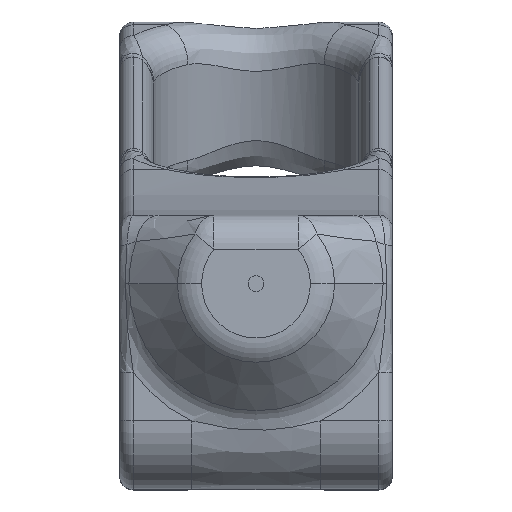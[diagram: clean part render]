
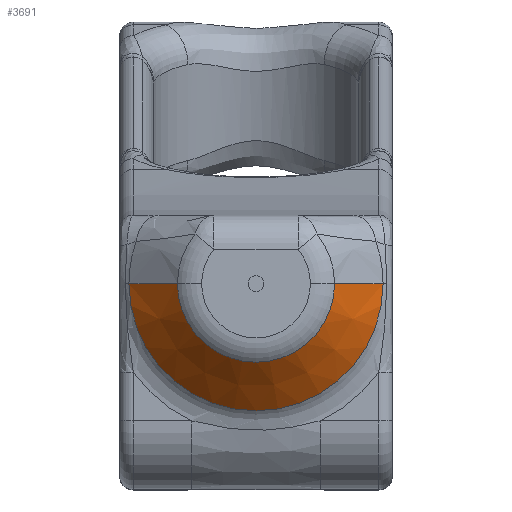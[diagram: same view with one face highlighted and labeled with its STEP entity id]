
A CAD part, top view. The second image highlights one B-rep face of the part: STEP entity #3691.
In plain terms, the highlighted conical face has half-angle 45 degrees and reference radius 5 mm.
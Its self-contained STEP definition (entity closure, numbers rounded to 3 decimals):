
#297 = EDGE_CURVE ( 'NONE', #1811, #1829, #3724, .T. ) ;
#663 = CARTESIAN_POINT ( 'NONE',  ( 0.681, 5., 18.232 ) ) ;
#1029 = DIRECTION ( 'NONE',  ( 0., 0., 1. ) ) ;
#1056 = EDGE_CURVE ( 'NONE', #2212, #2145, #3597, .T. ) ;
#1210 = DIRECTION ( 'NONE',  ( -1., 0., 0. ) ) ;
#1235 = EDGE_CURVE ( 'NONE', #2212, #1811, #2116, .T. ) ;
#1811 = VERTEX_POINT ( 'NONE', #3939 ) ;
#1829 = VERTEX_POINT ( 'NONE', #663 ) ;
#2077 = ORIENTED_EDGE ( 'NONE', *, *, #4556, .T. ) ;
#2116 = CIRCLE ( 'NONE', #2370, 5.732 ) ;
#2145 = VERTEX_POINT ( 'NONE', #4750 ) ;
#2212 = VERTEX_POINT ( 'NONE', #2391 ) ;
#2236 = CARTESIAN_POINT ( 'NONE',  ( 9.949, 5., 21.768 ) ) ;
#2284 = AXIS2_PLACEMENT_3D ( 'NONE', #3467, #1029, #3885 ) ;
#2370 = AXIS2_PLACEMENT_3D ( 'NONE', #2236, #5059, #2637 ) ;
#2391 = CARTESIAN_POINT ( 'NONE',  ( 15.681, 5., 21.768 ) ) ;
#2440 = DIRECTION ( 'NONE',  ( 0., 0., -1. ) ) ;
#2637 = DIRECTION ( 'NONE',  ( -1., 0., 0. ) ) ;
#3367 = FACE_OUTER_BOUND ( 'NONE', #3794, .T. ) ;
#3377 = DIRECTION ( 'NONE',  ( 0.707, 0., -0.707 ) ) ;
#3457 = VECTOR ( 'NONE', #3894, 1000. ) ;
#3467 = CARTESIAN_POINT ( 'NONE',  ( 9.949, 5., 18.232 ) ) ;
#3498 = CARTESIAN_POINT ( 'NONE',  ( 4.949, 5., 22.5 ) ) ;
#3597 = LINE ( 'NONE', #4970, #4784 ) ;
#3681 = ORIENTED_EDGE ( 'NONE', *, *, #1056, .F. ) ;
#3691 = ADVANCED_FACE ( 'NONE', ( #3367 ), #4189, .T. ) ;
#3724 = LINE ( 'NONE', #3498, #3457 ) ;
#3794 = EDGE_LOOP ( 'NONE', ( #3681, #4571, #4862, #2077 ) ) ;
#3811 = CIRCLE ( 'NONE', #2284, 9.268 ) ;
#3885 = DIRECTION ( 'NONE',  ( 1., 0., 0. ) ) ;
#3894 = DIRECTION ( 'NONE',  ( -0.707, 0., -0.707 ) ) ;
#3939 = CARTESIAN_POINT ( 'NONE',  ( 4.217, 5., 21.768 ) ) ;
#4189 = CONICAL_SURFACE ( 'NONE', #4787, 5., 0.785 ) ;
#4462 = CARTESIAN_POINT ( 'NONE',  ( 9.949, 5., 22.5 ) ) ;
#4556 = EDGE_CURVE ( 'NONE', #1829, #2145, #3811, .T. ) ;
#4571 = ORIENTED_EDGE ( 'NONE', *, *, #1235, .T. ) ;
#4750 = CARTESIAN_POINT ( 'NONE',  ( 19.217, 5., 18.232 ) ) ;
#4784 = VECTOR ( 'NONE', #3377, 1000. ) ;
#4787 = AXIS2_PLACEMENT_3D ( 'NONE', #4462, #2440, #1210 ) ;
#4862 = ORIENTED_EDGE ( 'NONE', *, *, #297, .T. ) ;
#4970 = CARTESIAN_POINT ( 'NONE',  ( 14.949, 5., 22.5 ) ) ;
#5059 = DIRECTION ( 'NONE',  ( 0., 0., -1. ) ) ;
